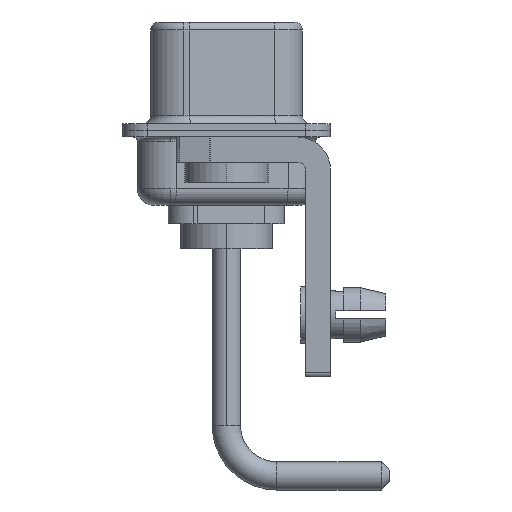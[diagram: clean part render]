
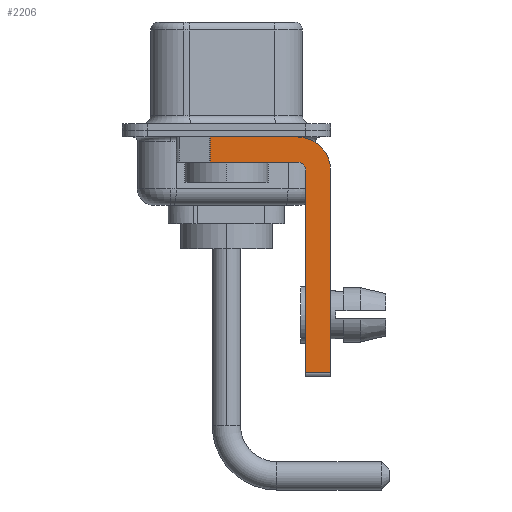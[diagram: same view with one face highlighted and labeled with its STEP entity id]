
A CAD part, left-side view. The second image highlights one B-rep face of the part: STEP entity #2206.
In plain terms, the highlighted planar face has unit normal (-1, 0, 0).
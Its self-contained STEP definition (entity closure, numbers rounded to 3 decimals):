
#19 = CARTESIAN_POINT ( 'NONE',  ( -2.9, 0.978, -1.9 ) ) ;
#89 = EDGE_CURVE ( 'NONE', #6244, #12003, #11933, .T. ) ;
#93 = CIRCLE ( 'NONE', #7466, 2. ) ;
#324 = VECTOR ( 'NONE', #15206, 1000. ) ;
#408 = LINE ( 'NONE', #15777, #13673 ) ;
#456 = EDGE_CURVE ( 'NONE', #7067, #13778, #8484, .T. ) ;
#883 = DIRECTION ( 'NONE',  ( 0., -1., 0. ) ) ;
#1336 = ORIENTED_EDGE ( 'NONE', *, *, #4543, .F. ) ;
#1422 = CARTESIAN_POINT ( 'NONE',  ( -2.9, -4.25, -2.4 ) ) ;
#1585 = ORIENTED_EDGE ( 'NONE', *, *, #13676, .F. ) ;
#2053 = VERTEX_POINT ( 'NONE', #8774 ) ;
#2176 = LINE ( 'NONE', #12632, #11862 ) ;
#2206 = ADVANCED_FACE ( 'NONE', ( #7921 ), #13176, .F. ) ;
#2366 = CARTESIAN_POINT ( 'NONE',  ( -2.9, -4.25, -1.9 ) ) ;
#2424 = DIRECTION ( 'NONE',  ( 0., 0., 1. ) ) ;
#2702 = CARTESIAN_POINT ( 'NONE',  ( -2.9, -4.75, -14.8 ) ) ;
#3072 = VECTOR ( 'NONE', #13150, 1000. ) ;
#3924 = DIRECTION ( 'NONE',  ( 0., 0., -1. ) ) ;
#4055 = EDGE_CURVE ( 'NONE', #8830, #13778, #408, .T. ) ;
#4062 = ORIENTED_EDGE ( 'NONE', *, *, #9738, .F. ) ;
#4212 = CARTESIAN_POINT ( 'NONE',  ( -2.9, -4.75, -14.55 ) ) ;
#4543 = EDGE_CURVE ( 'NONE', #12003, #6538, #11788, .T. ) ;
#5259 = CARTESIAN_POINT ( 'NONE',  ( -2.9, -4.25, -1.9 ) ) ;
#5630 = DIRECTION ( 'NONE',  ( 0., 0., -1. ) ) ;
#6244 = VERTEX_POINT ( 'NONE', #10114 ) ;
#6376 = CARTESIAN_POINT ( 'NONE',  ( -2.9, -6.25, -14.55 ) ) ;
#6538 = VERTEX_POINT ( 'NONE', #11864 ) ;
#6642 = DIRECTION ( 'NONE',  ( 1., 0., 0. ) ) ;
#7067 = VERTEX_POINT ( 'NONE', #4212 ) ;
#7086 = VECTOR ( 'NONE', #10497, 1000. ) ;
#7152 = VECTOR ( 'NONE', #7910, 1000. ) ;
#7258 = CARTESIAN_POINT ( 'NONE',  ( -2.9, -6.25, -2.4 ) ) ;
#7466 = AXIS2_PLACEMENT_3D ( 'NONE', #15347, #11718, #3924 ) ;
#7910 = DIRECTION ( 'NONE',  ( 0., 0., 1. ) ) ;
#7921 = FACE_OUTER_BOUND ( 'NONE', #13486, .T. ) ;
#8058 = ORIENTED_EDGE ( 'NONE', *, *, #4055, .F. ) ;
#8479 = ORIENTED_EDGE ( 'NONE', *, *, #456, .T. ) ;
#8484 = LINE ( 'NONE', #9773, #324 ) ;
#8774 = CARTESIAN_POINT ( 'NONE',  ( -2.9, 0.978, -0.4 ) ) ;
#8830 = VERTEX_POINT ( 'NONE', #7258 ) ;
#8881 = ORIENTED_EDGE ( 'NONE', *, *, #10121, .F. ) ;
#9092 = LINE ( 'NONE', #19, #3072 ) ;
#9738 = EDGE_CURVE ( 'NONE', #2053, #11397, #2176, .T. ) ;
#9773 = CARTESIAN_POINT ( 'NONE',  ( -2.9, -4.25, -14.55 ) ) ;
#10114 = CARTESIAN_POINT ( 'NONE',  ( -2.9, -4.75, -2.4 ) ) ;
#10121 = EDGE_CURVE ( 'NONE', #11397, #8830, #93, .T. ) ;
#10497 = DIRECTION ( 'NONE',  ( 0., 1., 0. ) ) ;
#10564 = DIRECTION ( 'NONE',  ( -1., 0., 0. ) ) ;
#10590 = DIRECTION ( 'NONE',  ( 0., 0., -1. ) ) ;
#10902 = CARTESIAN_POINT ( 'NONE',  ( -2.9, -4.25, -0.4 ) ) ;
#11397 = VERTEX_POINT ( 'NONE', #10902 ) ;
#11600 = CARTESIAN_POINT ( 'NONE',  ( -2.9, -4.25, -2.4 ) ) ;
#11620 = LINE ( 'NONE', #2702, #7152 ) ;
#11718 = DIRECTION ( 'NONE',  ( 1., 0., 0. ) ) ;
#11788 = LINE ( 'NONE', #5259, #7086 ) ;
#11862 = VECTOR ( 'NONE', #883, 1000. ) ;
#11864 = CARTESIAN_POINT ( 'NONE',  ( -2.9, 0.978, -1.9 ) ) ;
#11933 = CIRCLE ( 'NONE', #13312, 0.5 ) ;
#12003 = VERTEX_POINT ( 'NONE', #2366 ) ;
#12632 = CARTESIAN_POINT ( 'NONE',  ( -2.9, 3., -0.4 ) ) ;
#13150 = DIRECTION ( 'NONE',  ( 0., 0., -1. ) ) ;
#13176 = PLANE ( 'NONE',  #16351 ) ;
#13312 = AXIS2_PLACEMENT_3D ( 'NONE', #11600, #10564, #2424 ) ;
#13486 = EDGE_LOOP ( 'NONE', ( #4062, #14804, #1336, #16613, #1585, #8479, #8058, #8881 ) ) ;
#13673 = VECTOR ( 'NONE', #5630, 1000. ) ;
#13676 = EDGE_CURVE ( 'NONE', #7067, #6244, #11620, .T. ) ;
#13778 = VERTEX_POINT ( 'NONE', #6376 ) ;
#14804 = ORIENTED_EDGE ( 'NONE', *, *, #15692, .T. ) ;
#15206 = DIRECTION ( 'NONE',  ( 0., -1., 0. ) ) ;
#15347 = CARTESIAN_POINT ( 'NONE',  ( -2.9, -4.25, -2.4 ) ) ;
#15692 = EDGE_CURVE ( 'NONE', #2053, #6538, #9092, .T. ) ;
#15777 = CARTESIAN_POINT ( 'NONE',  ( -2.9, -6.25, -2.4 ) ) ;
#16351 = AXIS2_PLACEMENT_3D ( 'NONE', #1422, #6642, #10590 ) ;
#16613 = ORIENTED_EDGE ( 'NONE', *, *, #89, .F. ) ;
